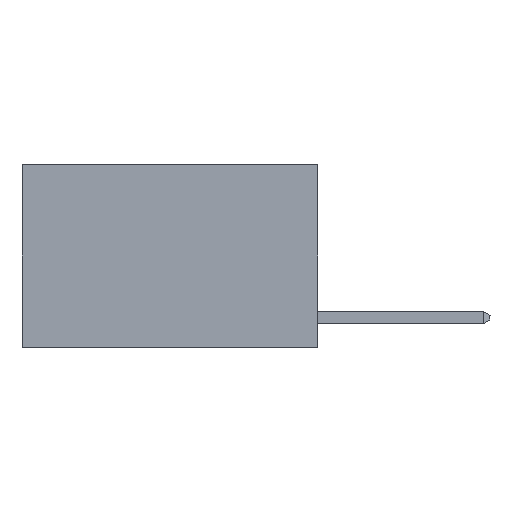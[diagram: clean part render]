
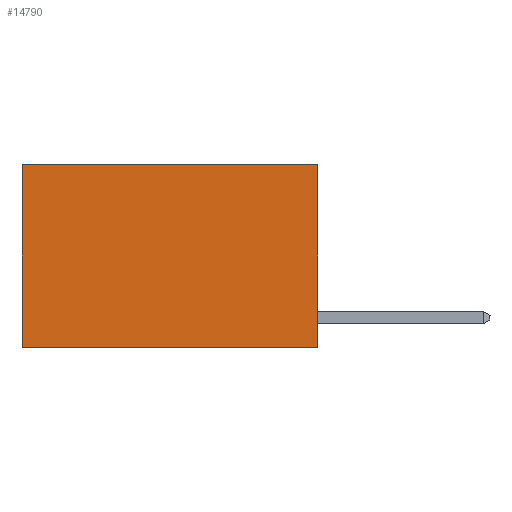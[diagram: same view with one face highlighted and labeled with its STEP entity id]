
A CAD part, left-side view. The second image highlights one B-rep face of the part: STEP entity #14790.
In plain terms, the highlighted planar face has unit normal (-1, 0, 0).
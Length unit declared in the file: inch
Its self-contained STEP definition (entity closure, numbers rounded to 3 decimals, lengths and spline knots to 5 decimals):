
#89 = LINE ( 'NONE', #12492, #14227 ) ;
#1097 = CARTESIAN_POINT ( 'NONE',  ( 0.2625, 0., 0. ) ) ;
#2420 = VERTEX_POINT ( 'NONE', #10898 ) ;
#2950 = PLANE ( 'NONE',  #13478 ) ;
#3635 = ORIENTED_EDGE ( 'NONE', *, *, #11717, .T. ) ;
#3722 = FACE_OUTER_BOUND ( 'NONE', #15171, .T. ) ;
#4296 = EDGE_CURVE ( 'NONE', #10163, #8730, #89, .T. ) ;
#4561 = DIRECTION ( 'NONE',  ( 0., 0., -1. ) ) ;
#4653 = EDGE_CURVE ( 'NONE', #6010, #10163, #6737, .T. ) ;
#5402 = DIRECTION ( 'NONE',  ( 0., 1., 0. ) ) ;
#6010 = VERTEX_POINT ( 'NONE', #7702 ) ;
#6737 = LINE ( 'NONE', #19157, #16799 ) ;
#6758 = DIRECTION ( 'NONE',  ( 0., 1., 0. ) ) ;
#7056 = VECTOR ( 'NONE', #10277, 39.37008 ) ;
#7702 = CARTESIAN_POINT ( 'NONE',  ( 0.2625, 0., 0. ) ) ;
#7948 = ORIENTED_EDGE ( 'NONE', *, *, #4653, .F. ) ;
#8730 = VERTEX_POINT ( 'NONE', #16887 ) ;
#8922 = VECTOR ( 'NONE', #6758, 39.37008 ) ;
#10163 = VERTEX_POINT ( 'NONE', #12599 ) ;
#10277 = DIRECTION ( 'NONE',  ( 0., 0., -1. ) ) ;
#10639 = ORIENTED_EDGE ( 'NONE', *, *, #17570, .T. ) ;
#10898 = CARTESIAN_POINT ( 'NONE',  ( 0.2625, 0.6, 0. ) ) ;
#11717 = EDGE_CURVE ( 'NONE', #2420, #8730, #16553, .T. ) ;
#12492 = CARTESIAN_POINT ( 'NONE',  ( 0.2625, 0., -0.37 ) ) ;
#12599 = CARTESIAN_POINT ( 'NONE',  ( 0.2625, 0., -0.37 ) ) ;
#12939 = LINE ( 'NONE', #1097, #8922 ) ;
#13478 = AXIS2_PLACEMENT_3D ( 'NONE', #21374, #21937, #18273 ) ;
#14061 = CARTESIAN_POINT ( 'NONE',  ( 0.2625, 0.6, 0. ) ) ;
#14227 = VECTOR ( 'NONE', #5402, 39.37008 ) ;
#14790 = ADVANCED_FACE ( 'NONE', ( #3722 ), #2950, .F. ) ;
#15171 = EDGE_LOOP ( 'NONE', ( #3635, #22498, #7948, #10639 ) ) ;
#16553 = LINE ( 'NONE', #14061, #7056 ) ;
#16799 = VECTOR ( 'NONE', #4561, 39.37008 ) ;
#16887 = CARTESIAN_POINT ( 'NONE',  ( 0.2625, 0.6, -0.37 ) ) ;
#17570 = EDGE_CURVE ( 'NONE', #6010, #2420, #12939, .T. ) ;
#18273 = DIRECTION ( 'NONE',  ( 0., 0., -1. ) ) ;
#19157 = CARTESIAN_POINT ( 'NONE',  ( 0.2625, 0., 0. ) ) ;
#21374 = CARTESIAN_POINT ( 'NONE',  ( 0.2625, 0., 0. ) ) ;
#21937 = DIRECTION ( 'NONE',  ( 1., 0., 0. ) ) ;
#22498 = ORIENTED_EDGE ( 'NONE', *, *, #4296, .F. ) ;
